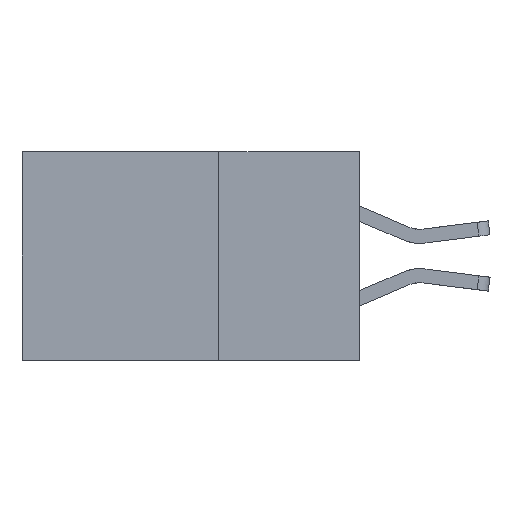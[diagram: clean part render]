
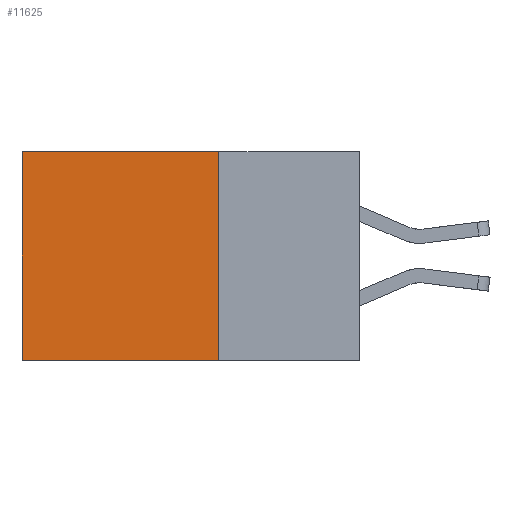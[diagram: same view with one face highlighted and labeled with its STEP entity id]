
A CAD part, left-side view. The second image highlights one B-rep face of the part: STEP entity #11625.
In plain terms, the highlighted planar face has unit normal (-1, 0, 0).
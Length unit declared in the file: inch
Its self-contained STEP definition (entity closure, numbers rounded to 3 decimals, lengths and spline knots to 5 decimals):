
#819 = DIRECTION ( 'NONE',  ( 0., 1., 0. ) ) ;
#1578 = VECTOR ( 'NONE', #10895, 39.37008 ) ;
#1594 = EDGE_CURVE ( 'NONE', #4887, #6387, #13164, .T. ) ;
#1759 = ORIENTED_EDGE ( 'NONE', *, *, #11318, .T. ) ;
#2759 = CARTESIAN_POINT ( 'NONE',  ( 0.2875, 0.25, 0. ) ) ;
#2822 = DIRECTION ( 'NONE',  ( 0., 1., 0. ) ) ;
#4119 = LINE ( 'NONE', #9584, #8327 ) ;
#4156 = FACE_OUTER_BOUND ( 'NONE', #9010, .T. ) ;
#4816 = CARTESIAN_POINT ( 'NONE',  ( 0.2875, 0.6, 0. ) ) ;
#4887 = VERTEX_POINT ( 'NONE', #14211 ) ;
#5530 = PLANE ( 'NONE',  #6830 ) ;
#5639 = DIRECTION ( 'NONE',  ( 0., 0., -1. ) ) ;
#6032 = VECTOR ( 'NONE', #819, 39.37008 ) ;
#6387 = VERTEX_POINT ( 'NONE', #12470 ) ;
#6830 = AXIS2_PLACEMENT_3D ( 'NONE', #12672, #12528, #5639 ) ;
#7107 = EDGE_CURVE ( 'NONE', #10240, #4887, #7743, .T. ) ;
#7743 = LINE ( 'NONE', #2759, #1578 ) ;
#8296 = VERTEX_POINT ( 'NONE', #4816 ) ;
#8327 = VECTOR ( 'NONE', #13168, 39.37008 ) ;
#9010 = EDGE_LOOP ( 'NONE', ( #14572, #11628, #11189, #1759 ) ) ;
#9584 = CARTESIAN_POINT ( 'NONE',  ( 0.2875, 0.6, 0. ) ) ;
#9760 = CARTESIAN_POINT ( 'NONE',  ( 0.2875, 0.25, 0. ) ) ;
#10155 = LINE ( 'NONE', #11009, #12543 ) ;
#10240 = VERTEX_POINT ( 'NONE', #9760 ) ;
#10895 = DIRECTION ( 'NONE',  ( 0., 0., -1. ) ) ;
#11009 = CARTESIAN_POINT ( 'NONE',  ( 0.2875, 0.25, 0. ) ) ;
#11189 = ORIENTED_EDGE ( 'NONE', *, *, #7107, .F. ) ;
#11218 = CARTESIAN_POINT ( 'NONE',  ( 0.2875, 0.25, -0.37 ) ) ;
#11318 = EDGE_CURVE ( 'NONE', #10240, #8296, #10155, .T. ) ;
#11625 = ADVANCED_FACE ( 'NONE', ( #4156 ), #5530, .F. ) ;
#11628 = ORIENTED_EDGE ( 'NONE', *, *, #1594, .F. ) ;
#12470 = CARTESIAN_POINT ( 'NONE',  ( 0.2875, 0.6, -0.37 ) ) ;
#12528 = DIRECTION ( 'NONE',  ( 1., 0., 0. ) ) ;
#12543 = VECTOR ( 'NONE', #2822, 39.37008 ) ;
#12672 = CARTESIAN_POINT ( 'NONE',  ( 0.2875, 0.25, 0. ) ) ;
#13164 = LINE ( 'NONE', #11218, #6032 ) ;
#13168 = DIRECTION ( 'NONE',  ( 0., 0., -1. ) ) ;
#13891 = EDGE_CURVE ( 'NONE', #8296, #6387, #4119, .T. ) ;
#14211 = CARTESIAN_POINT ( 'NONE',  ( 0.2875, 0.25, -0.37 ) ) ;
#14572 = ORIENTED_EDGE ( 'NONE', *, *, #13891, .T. ) ;
